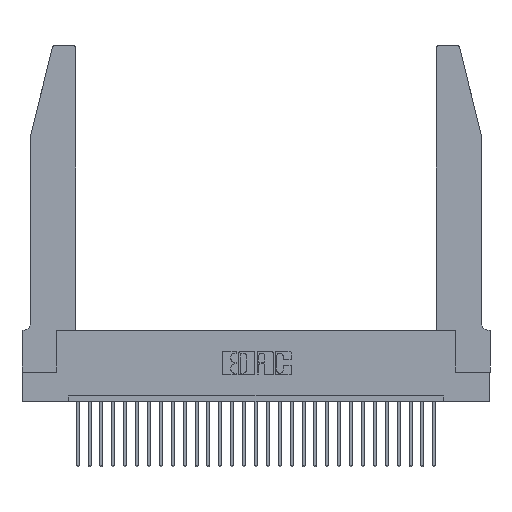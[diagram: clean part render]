
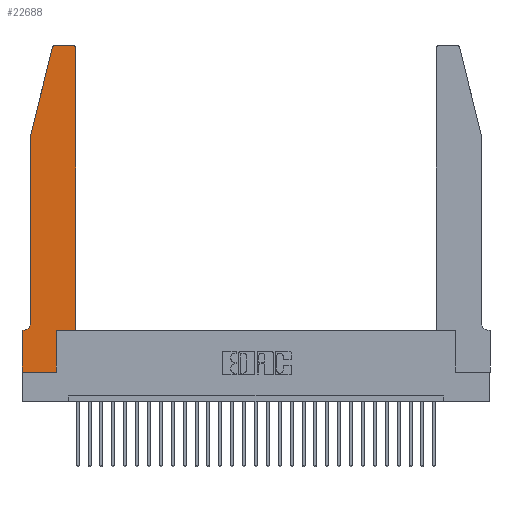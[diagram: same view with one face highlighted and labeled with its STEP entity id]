
A CAD part, top view. The second image highlights one B-rep face of the part: STEP entity #22688.
In plain terms, the highlighted planar face has unit normal (0, 0, 1).
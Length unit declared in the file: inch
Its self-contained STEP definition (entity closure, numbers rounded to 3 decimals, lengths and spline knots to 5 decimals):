
#659 = DIRECTION ( 'NONE',  ( 0., -1., 0. ) ) ;
#1141 = CARTESIAN_POINT ( 'NONE',  ( 0.0755, 0.42, 0.37 ) ) ;
#1396 = CARTESIAN_POINT ( 'NONE',  ( 0.0055, 0.42, 0.37 ) ) ;
#2228 = CIRCLE ( 'NONE', #4635, 0.07 ) ;
#2424 = AXIS2_PLACEMENT_3D ( 'NONE', #15561, #6388, #19873 ) ;
#2535 = CARTESIAN_POINT ( 'NONE',  ( 0.4505, 0.35, 0.37 ) ) ;
#2576 = VERTEX_POINT ( 'NONE', #29519 ) ;
#2631 = CARTESIAN_POINT ( 'NONE',  ( 0.2605, 2.75, 0.37 ) ) ;
#3322 = VERTEX_POINT ( 'NONE', #20944 ) ;
#3359 = EDGE_CURVE ( 'NONE', #11696, #27983, #5368, .T. ) ;
#3449 = DIRECTION ( 'NONE',  ( 0., 1., 0. ) ) ;
#3574 = EDGE_LOOP ( 'NONE', ( #14448, #5423, #10669, #10004, #11878, #10295, #20170, #14363, #16831, #26113, #22598, #11063 ) ) ;
#3699 = CARTESIAN_POINT ( 'NONE',  ( 0.4505, 0.35, 0.37 ) ) ;
#3723 = DIRECTION ( 'NONE',  ( -1., 0., 0. ) ) ;
#4539 = DIRECTION ( 'NONE',  ( 1., 0., 0. ) ) ;
#4635 = AXIS2_PLACEMENT_3D ( 'NONE', #1396, #17387, #3723 ) ;
#4682 = CARTESIAN_POINT ( 'NONE',  ( 0.0755, 2., 0.37 ) ) ;
#5225 = DIRECTION ( 'NONE',  ( -1., 0., 0. ) ) ;
#5358 = CARTESIAN_POINT ( 'NONE',  ( 0.0755, 0.35, 0.37 ) ) ;
#5368 = LINE ( 'NONE', #11962, #17861 ) ;
#5423 = ORIENTED_EDGE ( 'NONE', *, *, #14563, .T. ) ;
#5582 = LINE ( 'NONE', #18017, #28733 ) ;
#6001 = EDGE_CURVE ( 'NONE', #12103, #14077, #5582, .T. ) ;
#6388 = DIRECTION ( 'NONE',  ( 0., 0., 1. ) ) ;
#6701 = CARTESIAN_POINT ( 'NONE',  ( 0., 0., 0.37 ) ) ;
#7108 = LINE ( 'NONE', #26081, #24948 ) ;
#7933 = CIRCLE ( 'NONE', #16013, 0.03 ) ;
#8120 = FACE_OUTER_BOUND ( 'NONE', #3574, .T. ) ;
#8659 = AXIS2_PLACEMENT_3D ( 'NONE', #15607, #17905, #4539 ) ;
#8884 = DIRECTION ( 'NONE',  ( -0.239, -0.971, 0. ) ) ;
#9109 = VERTEX_POINT ( 'NONE', #11052 ) ;
#10004 = ORIENTED_EDGE ( 'NONE', *, *, #17256, .T. ) ;
#10295 = ORIENTED_EDGE ( 'NONE', *, *, #10638, .T. ) ;
#10638 = EDGE_CURVE ( 'NONE', #13185, #9109, #29551, .T. ) ;
#10669 = ORIENTED_EDGE ( 'NONE', *, *, #25775, .T. ) ;
#11052 = CARTESIAN_POINT ( 'NONE',  ( 0., 0.35, 0.37 ) ) ;
#11063 = ORIENTED_EDGE ( 'NONE', *, *, #15356, .T. ) ;
#11173 = CARTESIAN_POINT ( 'NONE',  ( 0., 0., 0.37 ) ) ;
#11696 = VERTEX_POINT ( 'NONE', #2535 ) ;
#11737 = VECTOR ( 'NONE', #11750, 39.37008 ) ;
#11750 = DIRECTION ( 'NONE',  ( 0., -1., 0. ) ) ;
#11878 = ORIENTED_EDGE ( 'NONE', *, *, #24916, .T. ) ;
#11962 = CARTESIAN_POINT ( 'NONE',  ( 0.4505, 0.35, 0.37 ) ) ;
#12103 = VERTEX_POINT ( 'NONE', #6701 ) ;
#12461 = VECTOR ( 'NONE', #14436, 39.37008 ) ;
#12691 = VERTEX_POINT ( 'NONE', #26704 ) ;
#12913 = CARTESIAN_POINT ( 'NONE',  ( 0.0055, 0.35, 0.37 ) ) ;
#12944 = CARTESIAN_POINT ( 'NONE',  ( 0.0755, 2., 0.37 ) ) ;
#13185 = VERTEX_POINT ( 'NONE', #12913 ) ;
#13590 = EDGE_CURVE ( 'NONE', #12691, #22406, #22607, .T. ) ;
#13798 = CARTESIAN_POINT ( 'NONE',  ( 0.284, 2.75, 0.37 ) ) ;
#14077 = VERTEX_POINT ( 'NONE', #27260 ) ;
#14363 = ORIENTED_EDGE ( 'NONE', *, *, #6001, .T. ) ;
#14436 = DIRECTION ( 'NONE',  ( -1., 0., 0. ) ) ;
#14448 = ORIENTED_EDGE ( 'NONE', *, *, #13590, .T. ) ;
#14563 = EDGE_CURVE ( 'NONE', #22406, #2576, #23673, .T. ) ;
#14803 = CARTESIAN_POINT ( 'NONE',  ( 0.4505, 2.72, 0.37 ) ) ;
#15356 = EDGE_CURVE ( 'NONE', #27983, #12691, #7933, .T. ) ;
#15561 = CARTESIAN_POINT ( 'NONE',  ( 0.284, 2.72, 0.37 ) ) ;
#15607 = CARTESIAN_POINT ( 'NONE',  ( 0., 0.35, 0.37 ) ) ;
#15610 = CARTESIAN_POINT ( 'NONE',  ( 0.0755, 2., 0.37 ) ) ;
#15736 = VECTOR ( 'NONE', #8884, 39.37008 ) ;
#16013 = AXIS2_PLACEMENT_3D ( 'NONE', #25307, #27591, #18224 ) ;
#16430 = LINE ( 'NONE', #3699, #17512 ) ;
#16831 = ORIENTED_EDGE ( 'NONE', *, *, #18135, .T. ) ;
#17256 = EDGE_CURVE ( 'NONE', #21552, #24043, #22172, .T. ) ;
#17387 = DIRECTION ( 'NONE',  ( 0., 0., -1. ) ) ;
#17491 = VECTOR ( 'NONE', #659, 39.37008 ) ;
#17512 = VECTOR ( 'NONE', #24251, 39.37008 ) ;
#17861 = VECTOR ( 'NONE', #27702, 39.37008 ) ;
#17905 = DIRECTION ( 'NONE',  ( 0., 0., 1. ) ) ;
#18017 = CARTESIAN_POINT ( 'NONE',  ( 0., 0., 0.37 ) ) ;
#18135 = EDGE_CURVE ( 'NONE', #14077, #3322, #7108, .T. ) ;
#18206 = PLANE ( 'NONE',  #8659 ) ;
#18224 = DIRECTION ( 'NONE',  ( 1., 0., 0. ) ) ;
#19873 = DIRECTION ( 'NONE',  ( 1., 0., 0. ) ) ;
#20170 = ORIENTED_EDGE ( 'NONE', *, *, #27728, .T. ) ;
#20944 = CARTESIAN_POINT ( 'NONE',  ( 0.2865, 0.35, 0.37 ) ) ;
#21552 = VERTEX_POINT ( 'NONE', #12944 ) ;
#22172 = LINE ( 'NONE', #4682, #17491 ) ;
#22406 = VERTEX_POINT ( 'NONE', #13798 ) ;
#22531 = LINE ( 'NONE', #15610, #15736 ) ;
#22598 = ORIENTED_EDGE ( 'NONE', *, *, #3359, .T. ) ;
#22607 = LINE ( 'NONE', #2631, #22974 ) ;
#22688 = ADVANCED_FACE ( 'NONE', ( #8120 ), #18206, .T. ) ;
#22974 = VECTOR ( 'NONE', #5225, 39.37008 ) ;
#23673 = CIRCLE ( 'NONE', #2424, 0.03 ) ;
#24043 = VERTEX_POINT ( 'NONE', #1141 ) ;
#24251 = DIRECTION ( 'NONE',  ( 1., 0., 0. ) ) ;
#24916 = EDGE_CURVE ( 'NONE', #24043, #13185, #2228, .T. ) ;
#24948 = VECTOR ( 'NONE', #3449, 39.37008 ) ;
#25307 = CARTESIAN_POINT ( 'NONE',  ( 0.4205, 2.72, 0.37 ) ) ;
#25775 = EDGE_CURVE ( 'NONE', #2576, #21552, #22531, .T. ) ;
#26081 = CARTESIAN_POINT ( 'NONE',  ( 0.2865, 0.35, 0.37 ) ) ;
#26113 = ORIENTED_EDGE ( 'NONE', *, *, #26770, .T. ) ;
#26704 = CARTESIAN_POINT ( 'NONE',  ( 0.4205, 2.75, 0.37 ) ) ;
#26770 = EDGE_CURVE ( 'NONE', #3322, #11696, #16430, .T. ) ;
#27045 = LINE ( 'NONE', #11173, #11737 ) ;
#27260 = CARTESIAN_POINT ( 'NONE',  ( 0.2865, 0., 0.37 ) ) ;
#27284 = DIRECTION ( 'NONE',  ( 1., 0., 0. ) ) ;
#27591 = DIRECTION ( 'NONE',  ( 0., 0., 1. ) ) ;
#27702 = DIRECTION ( 'NONE',  ( 0., 1., 0. ) ) ;
#27728 = EDGE_CURVE ( 'NONE', #9109, #12103, #27045, .T. ) ;
#27983 = VERTEX_POINT ( 'NONE', #14803 ) ;
#28733 = VECTOR ( 'NONE', #27284, 39.37008 ) ;
#29519 = CARTESIAN_POINT ( 'NONE',  ( 0.25487, 2.72718, 0.37 ) ) ;
#29551 = LINE ( 'NONE', #5358, #12461 ) ;
